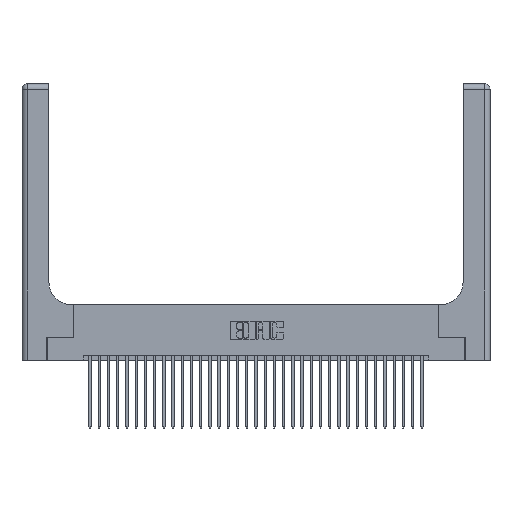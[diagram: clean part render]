
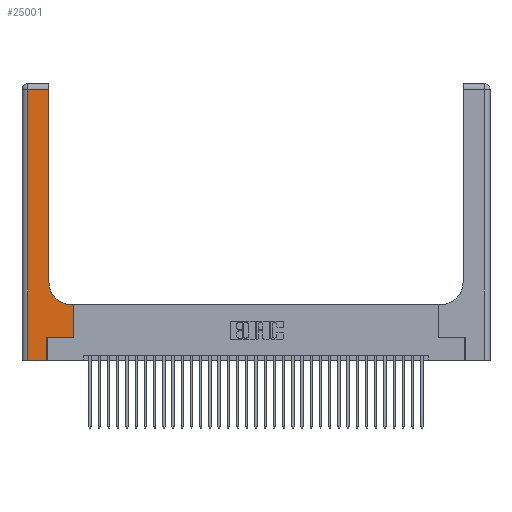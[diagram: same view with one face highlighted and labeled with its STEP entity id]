
A CAD part, top view. The second image highlights one B-rep face of the part: STEP entity #25001.
In plain terms, the highlighted planar face has unit normal (0, 0, 1).
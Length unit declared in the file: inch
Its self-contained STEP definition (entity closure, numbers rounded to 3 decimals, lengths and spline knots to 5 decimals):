
#98 = CARTESIAN_POINT ( 'NONE',  ( 0.06, 3., 0.37 ) ) ;
#569 = EDGE_CURVE ( 'NONE', #8228, #26112, #7767, .T. ) ;
#661 = CARTESIAN_POINT ( 'NONE',  ( 0.2915, 2.94, 0.37 ) ) ;
#778 = ORIENTED_EDGE ( 'NONE', *, *, #569, .T. ) ;
#1120 = VERTEX_POINT ( 'NONE', #10676 ) ;
#1850 = EDGE_CURVE ( 'NONE', #15647, #16916, #12651, .T. ) ;
#1922 = EDGE_CURVE ( 'NONE', #16916, #18061, #31619, .T. ) ;
#1977 = EDGE_CURVE ( 'NONE', #18061, #8228, #29919, .T. ) ;
#2849 = DIRECTION ( 'NONE',  ( 0., -1., 0. ) ) ;
#3203 = CARTESIAN_POINT ( 'NONE',  ( 0.2915, 3., 0.37 ) ) ;
#3600 = CARTESIAN_POINT ( 'NONE',  ( 0.269, 0.25, 0.37 ) ) ;
#4608 = PLANE ( 'NONE',  #19614 ) ;
#4999 = ORIENTED_EDGE ( 'NONE', *, *, #16221, .T. ) ;
#5334 = DIRECTION ( 'NONE',  ( 0., 1., 0. ) ) ;
#6335 = LINE ( 'NONE', #3203, #34176 ) ;
#6431 = CARTESIAN_POINT ( 'NONE',  ( 0.5415, 0.85, 0.37 ) ) ;
#6720 = EDGE_CURVE ( 'NONE', #27110, #25990, #19114, .T. ) ;
#7767 = LINE ( 'NONE', #8214, #28442 ) ;
#8214 = CARTESIAN_POINT ( 'NONE',  ( 0.269, 0., 0.37 ) ) ;
#8228 = VERTEX_POINT ( 'NONE', #27104 ) ;
#8891 = EDGE_CURVE ( 'NONE', #1120, #30391, #16625, .T. ) ;
#9118 = CARTESIAN_POINT ( 'NONE',  ( 0.2915, 0.85, 0.37 ) ) ;
#9159 = DIRECTION ( 'NONE',  ( 1., 0., 0. ) ) ;
#9392 = VECTOR ( 'NONE', #5334, 39.37008 ) ;
#9483 = EDGE_LOOP ( 'NONE', ( #10765, #18423, #29995, #24991, #778, #4999, #14193, #13037, #33475 ) ) ;
#9667 = VECTOR ( 'NONE', #30620, 39.37008 ) ;
#10037 = DIRECTION ( 'NONE',  ( 0., 0., -1. ) ) ;
#10633 = CARTESIAN_POINT ( 'NONE',  ( 0., 2.94, 0.37 ) ) ;
#10676 = CARTESIAN_POINT ( 'NONE',  ( 0.5585, 0.25, 0.37 ) ) ;
#10765 = ORIENTED_EDGE ( 'NONE', *, *, #22556, .T. ) ;
#11021 = CARTESIAN_POINT ( 'NONE',  ( 0.06, 0., 0.37 ) ) ;
#11334 = DIRECTION ( 'NONE',  ( 0., 1., 0. ) ) ;
#11689 = DIRECTION ( 'NONE',  ( -1., 0., 0. ) ) ;
#12208 = CARTESIAN_POINT ( 'NONE',  ( 0.269, 0.25, 0.37 ) ) ;
#12651 = LINE ( 'NONE', #10633, #33274 ) ;
#13037 = ORIENTED_EDGE ( 'NONE', *, *, #30026, .T. ) ;
#14193 = ORIENTED_EDGE ( 'NONE', *, *, #8891, .T. ) ;
#15404 = VECTOR ( 'NONE', #11689, 39.37008 ) ;
#15647 = VERTEX_POINT ( 'NONE', #661 ) ;
#16221 = EDGE_CURVE ( 'NONE', #26112, #1120, #18588, .T. ) ;
#16625 = LINE ( 'NONE', #24388, #9392 ) ;
#16916 = VERTEX_POINT ( 'NONE', #30663 ) ;
#18061 = VERTEX_POINT ( 'NONE', #11021 ) ;
#18423 = ORIENTED_EDGE ( 'NONE', *, *, #1850, .T. ) ;
#18588 = LINE ( 'NONE', #3600, #9667 ) ;
#19114 = CIRCLE ( 'NONE', #21127, 0.25 ) ;
#19295 = DIRECTION ( 'NONE',  ( 1., 0., 0. ) ) ;
#19614 = AXIS2_PLACEMENT_3D ( 'NONE', #26226, #10037, #28912 ) ;
#21127 = AXIS2_PLACEMENT_3D ( 'NONE', #6431, #25350, #9159 ) ;
#21745 = DIRECTION ( 'NONE',  ( 0., 1., 0. ) ) ;
#22022 = CARTESIAN_POINT ( 'NONE',  ( 0., 0., 0.37 ) ) ;
#22556 = EDGE_CURVE ( 'NONE', #25990, #15647, #6335, .T. ) ;
#23996 = FACE_OUTER_BOUND ( 'NONE', #9483, .T. ) ;
#24388 = CARTESIAN_POINT ( 'NONE',  ( 0.5585, 0.25, 0.37 ) ) ;
#24778 = CARTESIAN_POINT ( 'NONE',  ( 0.5415, 0.6, 0.37 ) ) ;
#24991 = ORIENTED_EDGE ( 'NONE', *, *, #1977, .T. ) ;
#25001 = ADVANCED_FACE ( 'NONE', ( #23996 ), #4608, .F. ) ;
#25350 = DIRECTION ( 'NONE',  ( 0., 0., -1. ) ) ;
#25990 = VERTEX_POINT ( 'NONE', #9118 ) ;
#26112 = VERTEX_POINT ( 'NONE', #12208 ) ;
#26226 = CARTESIAN_POINT ( 'NONE',  ( 0., 3., 0.37 ) ) ;
#27104 = CARTESIAN_POINT ( 'NONE',  ( 0.269, 0., 0.37 ) ) ;
#27110 = VERTEX_POINT ( 'NONE', #24778 ) ;
#27824 = CARTESIAN_POINT ( 'NONE',  ( 0.2915, 0.6, 0.37 ) ) ;
#28442 = VECTOR ( 'NONE', #21745, 39.37008 ) ;
#28860 = LINE ( 'NONE', #27824, #15404 ) ;
#28912 = DIRECTION ( 'NONE',  ( -1., 0., 0. ) ) ;
#29077 = VECTOR ( 'NONE', #19295, 39.37008 ) ;
#29526 = DIRECTION ( 'NONE',  ( -1., 0., 0. ) ) ;
#29919 = LINE ( 'NONE', #22022, #29077 ) ;
#29995 = ORIENTED_EDGE ( 'NONE', *, *, #1922, .T. ) ;
#30026 = EDGE_CURVE ( 'NONE', #30391, #27110, #28860, .T. ) ;
#30391 = VERTEX_POINT ( 'NONE', #34507 ) ;
#30620 = DIRECTION ( 'NONE',  ( 1., 0., 0. ) ) ;
#30663 = CARTESIAN_POINT ( 'NONE',  ( 0.06, 2.94, 0.37 ) ) ;
#31619 = LINE ( 'NONE', #98, #32453 ) ;
#32453 = VECTOR ( 'NONE', #2849, 39.37008 ) ;
#33274 = VECTOR ( 'NONE', #29526, 39.37008 ) ;
#33475 = ORIENTED_EDGE ( 'NONE', *, *, #6720, .T. ) ;
#34176 = VECTOR ( 'NONE', #11334, 39.37008 ) ;
#34507 = CARTESIAN_POINT ( 'NONE',  ( 0.5585, 0.6, 0.37 ) ) ;
